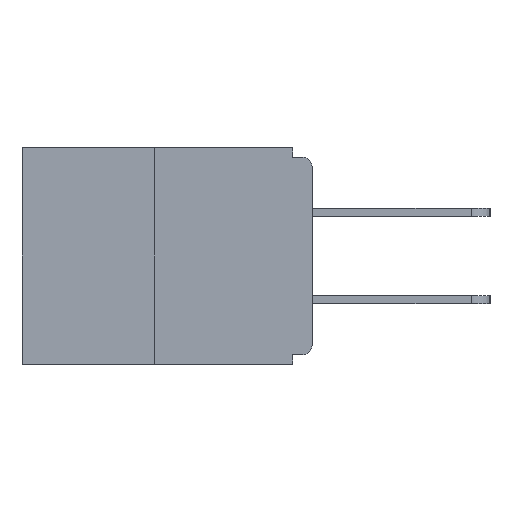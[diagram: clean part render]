
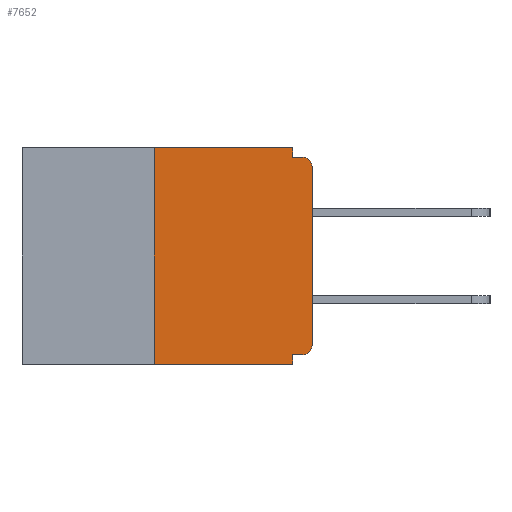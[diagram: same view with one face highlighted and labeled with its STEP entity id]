
A CAD part, left-side view. The second image highlights one B-rep face of the part: STEP entity #7652.
In plain terms, the highlighted planar face has unit normal (-1, 0, 0).
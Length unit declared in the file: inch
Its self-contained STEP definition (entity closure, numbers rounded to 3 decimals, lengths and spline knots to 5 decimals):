
#344 = CARTESIAN_POINT ( 'NONE',  ( 0., 0., 0. ) ) ;
#1091 = DIRECTION ( 'NONE',  ( 0., 0., -1. ) ) ;
#1376 = EDGE_LOOP ( 'NONE', ( #15453, #26083, #6305, #8317, #17817, #21829, #17845, #18187, #17344, #21215 ) ) ;
#2195 = CARTESIAN_POINT ( 'NONE',  ( 0., 0., -0.313 ) ) ;
#2614 = VECTOR ( 'NONE', #4850, 39.37008 ) ;
#2706 = VECTOR ( 'NONE', #28726, 39.37008 ) ;
#3658 = DIRECTION ( 'NONE',  ( 0., 0., -1. ) ) ;
#3660 = CARTESIAN_POINT ( 'NONE',  ( 0., 0.031, -0.015 ) ) ;
#4104 = VERTEX_POINT ( 'NONE', #23138 ) ;
#4507 = LINE ( 'NONE', #7835, #2706 ) ;
#4839 = VERTEX_POINT ( 'NONE', #9361 ) ;
#4850 = DIRECTION ( 'NONE',  ( 0., 0., 1. ) ) ;
#6305 = ORIENTED_EDGE ( 'NONE', *, *, #26844, .T. ) ;
#6704 = VECTOR ( 'NONE', #29150, 39.37008 ) ;
#7652 = ADVANCED_FACE ( 'NONE', ( #9492 ), #15437, .F. ) ;
#7656 = VECTOR ( 'NONE', #20792, 39.37008 ) ;
#7835 = CARTESIAN_POINT ( 'NONE',  ( 0., 0.46, 0. ) ) ;
#8161 = LINE ( 'NONE', #24664, #6704 ) ;
#8310 = CIRCLE ( 'NONE', #28446, 0.015 ) ;
#8317 = ORIENTED_EDGE ( 'NONE', *, *, #20813, .F. ) ;
#8701 = CARTESIAN_POINT ( 'NONE',  ( 0., 0.015, -0.328 ) ) ;
#8932 = VERTEX_POINT ( 'NONE', #2195 ) ;
#9263 = CARTESIAN_POINT ( 'NONE',  ( 0., 0.031, -0.343 ) ) ;
#9361 = CARTESIAN_POINT ( 'NONE',  ( 0., 0.015, -0.015 ) ) ;
#9386 = CARTESIAN_POINT ( 'NONE',  ( 0., 0.46, -0.343 ) ) ;
#9492 = FACE_OUTER_BOUND ( 'NONE', #1376, .T. ) ;
#10098 = AXIS2_PLACEMENT_3D ( 'NONE', #29181, #22204, #3658 ) ;
#10505 = CARTESIAN_POINT ( 'NONE',  ( 0., 0.031, -0.343 ) ) ;
#11538 = VERTEX_POINT ( 'NONE', #18015 ) ;
#11860 = AXIS2_PLACEMENT_3D ( 'NONE', #16380, #21072, #16573 ) ;
#12132 = VECTOR ( 'NONE', #1091, 39.37008 ) ;
#12750 = LINE ( 'NONE', #9386, #27707 ) ;
#13436 = LINE ( 'NONE', #21230, #28377 ) ;
#13860 = CARTESIAN_POINT ( 'NONE',  ( 0., 0.25, 0. ) ) ;
#14915 = CARTESIAN_POINT ( 'NONE',  ( 0., 0., -0.03 ) ) ;
#15295 = LINE ( 'NONE', #16505, #2614 ) ;
#15437 = PLANE ( 'NONE',  #11860 ) ;
#15453 = ORIENTED_EDGE ( 'NONE', *, *, #17974, .F. ) ;
#15936 = CARTESIAN_POINT ( 'NONE',  ( 0., 0.015, -0.03 ) ) ;
#16210 = CARTESIAN_POINT ( 'NONE',  ( 0., 0.031, 0. ) ) ;
#16380 = CARTESIAN_POINT ( 'NONE',  ( 0., 0.46, 0. ) ) ;
#16505 = CARTESIAN_POINT ( 'NONE',  ( 0., 0.25, 0. ) ) ;
#16573 = DIRECTION ( 'NONE',  ( 0., 0., -1. ) ) ;
#16995 = VERTEX_POINT ( 'NONE', #9263 ) ;
#17344 = ORIENTED_EDGE ( 'NONE', *, *, #24200, .F. ) ;
#17817 = ORIENTED_EDGE ( 'NONE', *, *, #20825, .F. ) ;
#17845 = ORIENTED_EDGE ( 'NONE', *, *, #22301, .T. ) ;
#17974 = EDGE_CURVE ( 'NONE', #25282, #11538, #4507, .T. ) ;
#18015 = CARTESIAN_POINT ( 'NONE',  ( 0., 0.031, 0. ) ) ;
#18187 = ORIENTED_EDGE ( 'NONE', *, *, #24749, .T. ) ;
#18798 = DIRECTION ( 'NONE',  ( 0., -1., 0. ) ) ;
#19047 = LINE ( 'NONE', #10505, #12132 ) ;
#19296 = CIRCLE ( 'NONE', #10098, 0.015 ) ;
#19714 = EDGE_CURVE ( 'NONE', #4104, #25282, #15295, .T. ) ;
#19717 = EDGE_CURVE ( 'NONE', #11538, #24986, #26639, .T. ) ;
#20792 = DIRECTION ( 'NONE',  ( 0., 0., -1. ) ) ;
#20813 = EDGE_CURVE ( 'NONE', #23259, #16995, #19047, .T. ) ;
#20825 = EDGE_CURVE ( 'NONE', #26565, #23259, #8161, .T. ) ;
#21072 = DIRECTION ( 'NONE',  ( 1., 0., 0. ) ) ;
#21215 = ORIENTED_EDGE ( 'NONE', *, *, #19717, .F. ) ;
#21230 = CARTESIAN_POINT ( 'NONE',  ( 0., 0., -0.015 ) ) ;
#21829 = ORIENTED_EDGE ( 'NONE', *, *, #26585, .T. ) ;
#22204 = DIRECTION ( 'NONE',  ( -1., 0., 0. ) ) ;
#22301 = EDGE_CURVE ( 'NONE', #8932, #29682, #25920, .T. ) ;
#22864 = DIRECTION ( 'NONE',  ( 0., 0., -1. ) ) ;
#23138 = CARTESIAN_POINT ( 'NONE',  ( 0., 0.25, -0.343 ) ) ;
#23259 = VERTEX_POINT ( 'NONE', #29797 ) ;
#24200 = EDGE_CURVE ( 'NONE', #24986, #4839, #13436, .T. ) ;
#24664 = CARTESIAN_POINT ( 'NONE',  ( 0., 0., -0.328 ) ) ;
#24749 = EDGE_CURVE ( 'NONE', #29682, #4839, #8310, .T. ) ;
#24986 = VERTEX_POINT ( 'NONE', #3660 ) ;
#25194 = VECTOR ( 'NONE', #25847, 39.37008 ) ;
#25282 = VERTEX_POINT ( 'NONE', #13860 ) ;
#25847 = DIRECTION ( 'NONE',  ( 0., 0., 1. ) ) ;
#25920 = LINE ( 'NONE', #344, #25194 ) ;
#26083 = ORIENTED_EDGE ( 'NONE', *, *, #19714, .F. ) ;
#26565 = VERTEX_POINT ( 'NONE', #8701 ) ;
#26585 = EDGE_CURVE ( 'NONE', #26565, #8932, #19296, .T. ) ;
#26639 = LINE ( 'NONE', #16210, #7656 ) ;
#26844 = EDGE_CURVE ( 'NONE', #4104, #16995, #12750, .T. ) ;
#27707 = VECTOR ( 'NONE', #28124, 39.37008 ) ;
#27872 = DIRECTION ( 'NONE',  ( -1., 0., 0. ) ) ;
#28124 = DIRECTION ( 'NONE',  ( 0., -1., 0. ) ) ;
#28377 = VECTOR ( 'NONE', #18798, 39.37008 ) ;
#28446 = AXIS2_PLACEMENT_3D ( 'NONE', #15936, #27872, #22864 ) ;
#28726 = DIRECTION ( 'NONE',  ( 0., -1., 0. ) ) ;
#29150 = DIRECTION ( 'NONE',  ( 0., 1., 0. ) ) ;
#29181 = CARTESIAN_POINT ( 'NONE',  ( 0., 0.015, -0.313 ) ) ;
#29682 = VERTEX_POINT ( 'NONE', #14915 ) ;
#29797 = CARTESIAN_POINT ( 'NONE',  ( 0., 0.031, -0.328 ) ) ;
